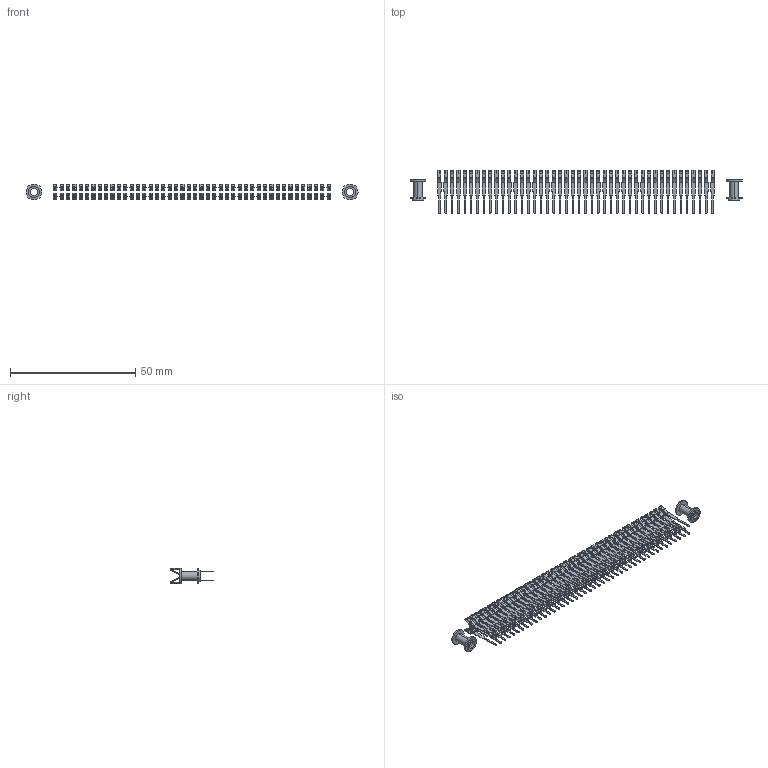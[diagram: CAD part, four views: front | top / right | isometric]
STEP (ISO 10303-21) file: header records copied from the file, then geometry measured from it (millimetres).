
FILE_DESCRIPTION (( 'STEP AP203' ), '1' );
FILE_NAME ('341-088-521-203.STEP', '2018-08-07T23:31:55', ( '' ), ( '' ), 'SwSTEP 2.0', 'SolidWorks 2016', '' );
FILE_SCHEMA (( 'CONFIG_CONTROL_DESIGN' ));
Length unit declared in the file: inch
Products named in the file (4): 341 Part_.156 (3.96) Dia Mounting Holes; 341-292-001_341-292-121; 345-250-002_345-250-002-102; 341-088-521-203
Assembly tree (91 placements, depth 2):
  341-088-521-203
    341 Part_.156 (3.96) Dia Mounting Holes
    341-292-001_341-292-121  x88
    345-250-002_345-250-002-102  x2
Bounding box: 132.72 x 17.2 x 6.35 mm (x, y, z)
Volume: 803.7 mm3; surface area: 6554.1 mm2
Topology: 90 solids, 90 shells, 4438 faces, 12924 edges, 8496 vertices
Faces by surface type: plane 2562, cylinder 1868, cone 8
Entity records: 54048 total; most frequent: CARTESIAN_POINT 8965, ORIENTED_EDGE 8900, DIRECTION 8714, EDGE_CURVE 4450, VECTOR 3588, LINE 3588, VERTEX_POINT 2814, AXIS2_PLACEMENT_3D 2563
